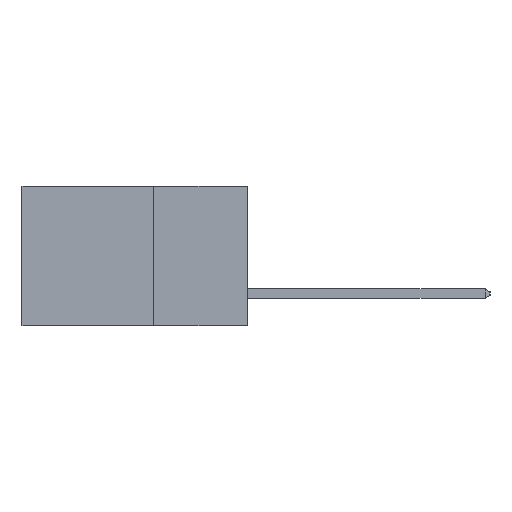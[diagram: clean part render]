
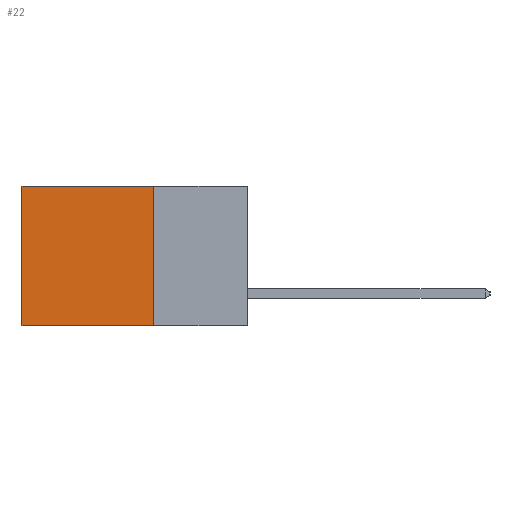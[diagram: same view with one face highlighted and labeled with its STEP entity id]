
A CAD part, left-side view. The second image highlights one B-rep face of the part: STEP entity #22.
In plain terms, the highlighted planar face has unit normal (-1, 0, 0).
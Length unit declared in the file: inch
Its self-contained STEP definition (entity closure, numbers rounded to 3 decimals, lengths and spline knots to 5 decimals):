
#22 = ADVANCED_FACE ( 'NONE', ( #19841 ), #20930, .F. ) ;
#563 = LINE ( 'NONE', #14086, #21577 ) ;
#2879 = EDGE_CURVE ( 'NONE', #24752, #18099, #563, .T. ) ;
#4250 = LINE ( 'NONE', #9607, #7764 ) ;
#7130 = VECTOR ( 'NONE', #17270, 39.37008 ) ;
#7764 = VECTOR ( 'NONE', #25526, 39.37008 ) ;
#8724 = VERTEX_POINT ( 'NONE', #18465 ) ;
#9607 = CARTESIAN_POINT ( 'NONE',  ( 0.2615, 0.6, -0.37 ) ) ;
#9922 = AXIS2_PLACEMENT_3D ( 'NONE', #11262, #10941, #14269 ) ;
#10008 = ORIENTED_EDGE ( 'NONE', *, *, #15696, .T. ) ;
#10941 = DIRECTION ( 'NONE',  ( 1., 0., 0. ) ) ;
#11262 = CARTESIAN_POINT ( 'NONE',  ( 0.2615, 0.25, -0.37 ) ) ;
#13587 = DIRECTION ( 'NONE',  ( 0., 1., 0. ) ) ;
#14086 = CARTESIAN_POINT ( 'NONE',  ( 0.2615, 0.25, -0.37 ) ) ;
#14269 = DIRECTION ( 'NONE',  ( 0., 0., -1. ) ) ;
#15255 = DIRECTION ( 'NONE',  ( 0., 1., 0. ) ) ;
#15477 = CARTESIAN_POINT ( 'NONE',  ( 0.2615, 0.6, -0.37 ) ) ;
#15696 = EDGE_CURVE ( 'NONE', #22537, #8724, #22053, .T. ) ;
#16035 = ORIENTED_EDGE ( 'NONE', *, *, #2879, .F. ) ;
#16828 = VECTOR ( 'NONE', #15255, 39.37008 ) ;
#17270 = DIRECTION ( 'NONE',  ( 0., 0., -1. ) ) ;
#18099 = VERTEX_POINT ( 'NONE', #15477 ) ;
#18465 = CARTESIAN_POINT ( 'NONE',  ( 0.2615, 0.6, 0. ) ) ;
#19260 = CARTESIAN_POINT ( 'NONE',  ( 0.2615, 0.25, -0.37 ) ) ;
#19627 = CARTESIAN_POINT ( 'NONE',  ( 0.2615, 0.25, -0.37 ) ) ;
#19841 = FACE_OUTER_BOUND ( 'NONE', #19885, .T. ) ;
#19885 = EDGE_LOOP ( 'NONE', ( #22070, #16035, #20426, #10008 ) ) ;
#20426 = ORIENTED_EDGE ( 'NONE', *, *, #23430, .F. ) ;
#20930 = PLANE ( 'NONE',  #9922 ) ;
#20977 = EDGE_CURVE ( 'NONE', #8724, #18099, #4250, .T. ) ;
#21577 = VECTOR ( 'NONE', #13587, 39.37008 ) ;
#22053 = LINE ( 'NONE', #23099, #16828 ) ;
#22070 = ORIENTED_EDGE ( 'NONE', *, *, #20977, .T. ) ;
#22537 = VERTEX_POINT ( 'NONE', #24450 ) ;
#23099 = CARTESIAN_POINT ( 'NONE',  ( 0.2615, 0.25, 0. ) ) ;
#23430 = EDGE_CURVE ( 'NONE', #22537, #24752, #24395, .T. ) ;
#24395 = LINE ( 'NONE', #19260, #7130 ) ;
#24450 = CARTESIAN_POINT ( 'NONE',  ( 0.2615, 0.25, 0. ) ) ;
#24752 = VERTEX_POINT ( 'NONE', #19627 ) ;
#25526 = DIRECTION ( 'NONE',  ( 0., 0., -1. ) ) ;
